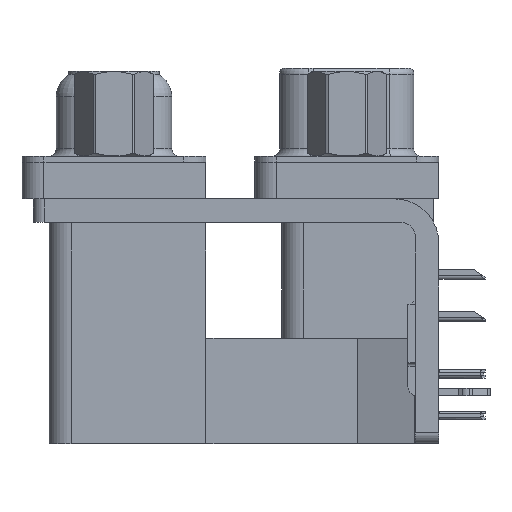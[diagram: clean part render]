
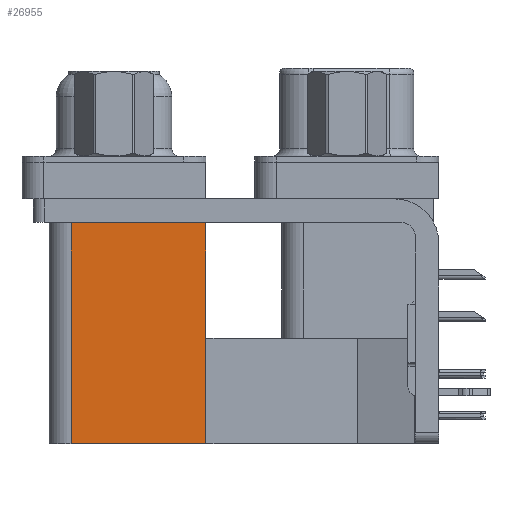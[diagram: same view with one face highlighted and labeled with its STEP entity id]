
A CAD part, left-side view. The second image highlights one B-rep face of the part: STEP entity #26955.
In plain terms, the highlighted planar face has unit normal (-1, 0, 0).
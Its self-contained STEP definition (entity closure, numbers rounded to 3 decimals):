
#1828 = EDGE_CURVE ( 'NONE', #42327, #34007, #3380, .T. ) ;
#1988 = DIRECTION ( 'NONE',  ( 0., 1., 0. ) ) ;
#3380 = LINE ( 'NONE', #30498, #23641 ) ;
#5601 = ORIENTED_EDGE ( 'NONE', *, *, #8558, .T. ) ;
#5759 = FACE_OUTER_BOUND ( 'NONE', #20670, .T. ) ;
#6145 = LINE ( 'NONE', #25947, #13318 ) ;
#6709 = LINE ( 'NONE', #30500, #26089 ) ;
#6853 = CARTESIAN_POINT ( 'NONE',  ( 3.79, 9.6, -19.2 ) ) ;
#8558 = EDGE_CURVE ( 'NONE', #42327, #20575, #30570, .T. ) ;
#9245 = ORIENTED_EDGE ( 'NONE', *, *, #1828, .F. ) ;
#9688 = DIRECTION ( 'NONE',  ( 0., 0., 1. ) ) ;
#10939 = VECTOR ( 'NONE', #9688, 1000. ) ;
#12395 = DIRECTION ( 'NONE',  ( 0., 1., 0. ) ) ;
#12506 = VERTEX_POINT ( 'NONE', #21076 ) ;
#13318 = VECTOR ( 'NONE', #12395, 1000. ) ;
#13606 = DIRECTION ( 'NONE',  ( 0., 1., 0. ) ) ;
#15334 = PLANE ( 'NONE',  #32958 ) ;
#16983 = ORIENTED_EDGE ( 'NONE', *, *, #33156, .F. ) ;
#19258 = EDGE_CURVE ( 'NONE', #20575, #12506, #6145, .T. ) ;
#19941 = CARTESIAN_POINT ( 'NONE',  ( 3.79, 18.8, -19.2 ) ) ;
#20347 = CARTESIAN_POINT ( 'NONE',  ( 3.79, 9.6, -19.2 ) ) ;
#20575 = VERTEX_POINT ( 'NONE', #22995 ) ;
#20670 = EDGE_LOOP ( 'NONE', ( #38859, #16983, #9245, #5601 ) ) ;
#21076 = CARTESIAN_POINT ( 'NONE',  ( 3.79, 18.8, -2.5 ) ) ;
#22995 = CARTESIAN_POINT ( 'NONE',  ( 3.79, 9.6, -2.5 ) ) ;
#23641 = VECTOR ( 'NONE', #13606, 1000. ) ;
#25947 = CARTESIAN_POINT ( 'NONE',  ( 3.79, 9.6, -2.5 ) ) ;
#26089 = VECTOR ( 'NONE', #30942, 1000. ) ;
#26955 = ADVANCED_FACE ( 'NONE', ( #5759 ), #15334, .F. ) ;
#29755 = DIRECTION ( 'NONE',  ( 1., 0., 0. ) ) ;
#30498 = CARTESIAN_POINT ( 'NONE',  ( 3.79, 9.6, -19.2 ) ) ;
#30500 = CARTESIAN_POINT ( 'NONE',  ( 3.79, 18.8, -19.2 ) ) ;
#30570 = LINE ( 'NONE', #20347, #10939 ) ;
#30942 = DIRECTION ( 'NONE',  ( 0., 0., 1. ) ) ;
#32861 = CARTESIAN_POINT ( 'NONE',  ( 3.79, 9.6, -19.2 ) ) ;
#32958 = AXIS2_PLACEMENT_3D ( 'NONE', #32861, #29755, #1988 ) ;
#33156 = EDGE_CURVE ( 'NONE', #34007, #12506, #6709, .T. ) ;
#34007 = VERTEX_POINT ( 'NONE', #19941 ) ;
#38859 = ORIENTED_EDGE ( 'NONE', *, *, #19258, .T. ) ;
#42327 = VERTEX_POINT ( 'NONE', #6853 ) ;
